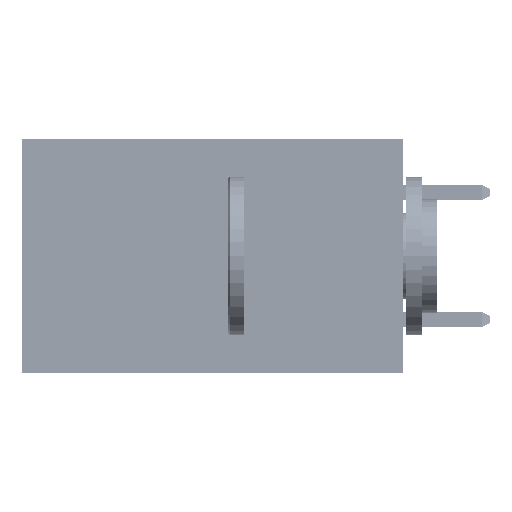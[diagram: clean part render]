
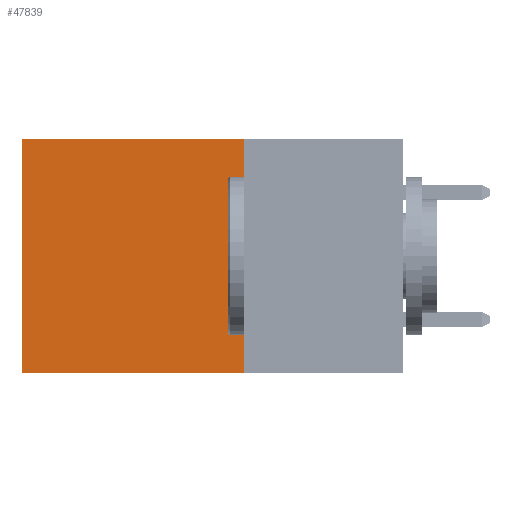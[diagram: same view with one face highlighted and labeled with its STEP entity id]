
A CAD part, left-side view. The second image highlights one B-rep face of the part: STEP entity #47839.
In plain terms, the highlighted planar face has unit normal (-1, 0, 0).
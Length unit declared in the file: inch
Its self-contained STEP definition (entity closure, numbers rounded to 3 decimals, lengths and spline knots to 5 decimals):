
#1254 = CARTESIAN_POINT ( 'NONE',  ( 0.2875, 0.25, 0. ) ) ;
#4194 = EDGE_CURVE ( 'NONE', #7432, #9571, #29324, .T. ) ;
#5217 = DIRECTION ( 'NONE',  ( 1., 0., 0. ) ) ;
#7432 = VERTEX_POINT ( 'NONE', #26147 ) ;
#9571 = VERTEX_POINT ( 'NONE', #33009 ) ;
#10067 = ORIENTED_EDGE ( 'NONE', *, *, #44031, .T. ) ;
#10467 = DIRECTION ( 'NONE',  ( 0., 0., -1. ) ) ;
#12198 = DIRECTION ( 'NONE',  ( 0., 0., -1. ) ) ;
#14469 = DIRECTION ( 'NONE',  ( 0., 1., 0. ) ) ;
#16855 = VECTOR ( 'NONE', #18992, 39.37008 ) ;
#18725 = FACE_OUTER_BOUND ( 'NONE', #47354, .T. ) ;
#18992 = DIRECTION ( 'NONE',  ( 0., 1., 0. ) ) ;
#20179 = PLANE ( 'NONE',  #32481 ) ;
#21732 = CARTESIAN_POINT ( 'NONE',  ( 0.2875, 0.6, -0.37 ) ) ;
#21921 = EDGE_CURVE ( 'NONE', #7432, #40325, #45086, .T. ) ;
#22002 = ORIENTED_EDGE ( 'NONE', *, *, #4194, .F. ) ;
#22118 = CARTESIAN_POINT ( 'NONE',  ( 0.2875, 0.6, 0. ) ) ;
#23660 = EDGE_CURVE ( 'NONE', #9571, #35417, #26010, .T. ) ;
#26010 = LINE ( 'NONE', #34570, #16855 ) ;
#26147 = CARTESIAN_POINT ( 'NONE',  ( 0.2875, 0.25, 0. ) ) ;
#26852 = LINE ( 'NONE', #41525, #31154 ) ;
#29324 = LINE ( 'NONE', #35719, #34250 ) ;
#29850 = CARTESIAN_POINT ( 'NONE',  ( 0.2875, 0.25, 0. ) ) ;
#31154 = VECTOR ( 'NONE', #10467, 39.37008 ) ;
#32481 = AXIS2_PLACEMENT_3D ( 'NONE', #1254, #5217, #12198 ) ;
#32916 = VECTOR ( 'NONE', #14469, 39.37008 ) ;
#33009 = CARTESIAN_POINT ( 'NONE',  ( 0.2875, 0.25, -0.37 ) ) ;
#34250 = VECTOR ( 'NONE', #43061, 39.37008 ) ;
#34570 = CARTESIAN_POINT ( 'NONE',  ( 0.2875, 0.25, -0.37 ) ) ;
#35417 = VERTEX_POINT ( 'NONE', #21732 ) ;
#35566 = ORIENTED_EDGE ( 'NONE', *, *, #23660, .F. ) ;
#35719 = CARTESIAN_POINT ( 'NONE',  ( 0.2875, 0.25, 0. ) ) ;
#40325 = VERTEX_POINT ( 'NONE', #22118 ) ;
#41525 = CARTESIAN_POINT ( 'NONE',  ( 0.2875, 0.6, 0. ) ) ;
#42565 = ORIENTED_EDGE ( 'NONE', *, *, #21921, .T. ) ;
#43061 = DIRECTION ( 'NONE',  ( 0., 0., -1. ) ) ;
#44031 = EDGE_CURVE ( 'NONE', #40325, #35417, #26852, .T. ) ;
#45086 = LINE ( 'NONE', #29850, #32916 ) ;
#47354 = EDGE_LOOP ( 'NONE', ( #10067, #35566, #22002, #42565 ) ) ;
#47839 = ADVANCED_FACE ( 'NONE', ( #18725 ), #20179, .F. ) ;
